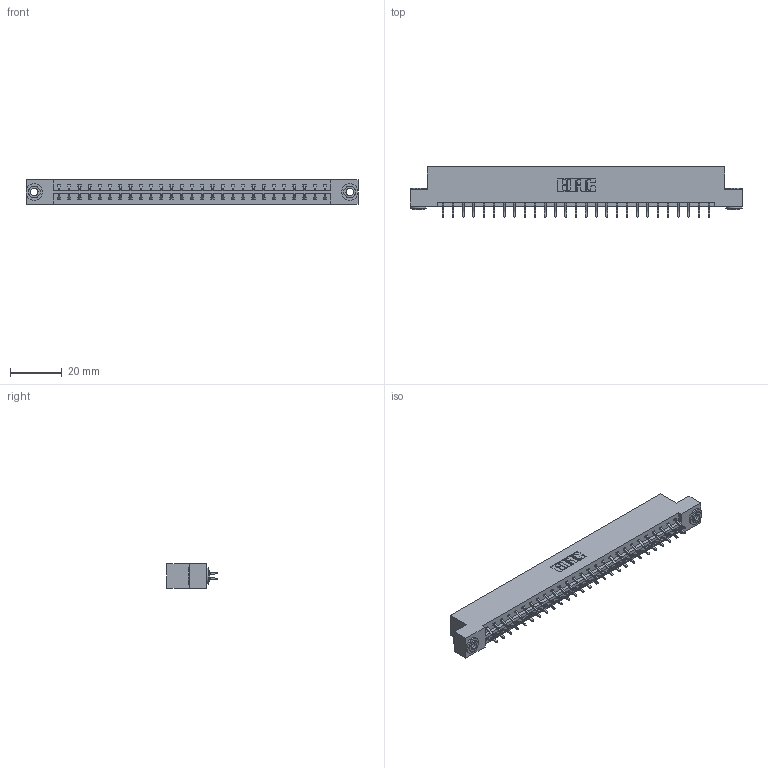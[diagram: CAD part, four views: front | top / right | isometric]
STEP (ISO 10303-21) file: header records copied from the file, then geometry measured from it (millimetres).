
FILE_DESCRIPTION (( 'STEP AP203' ), '1' );
FILE_NAME ('833-054-556-203.STEP', '2020-06-04T21:29:43', ( '' ), ( '' ), 'SwSTEP 2.0', 'SolidWorks 2020', '' );
FILE_SCHEMA (( 'CONFIG_CONTROL_DESIGN' ));
Length unit declared in the file: inch
Products named in the file (4): 345-292-001_556 Tail; 345-250-002_345-250-002-102; 833 Part_Flush - .156 Dia - TH; 833-054-556-203
Assembly tree (57 placements, depth 2):
  833-054-556-203
    833 Part_Flush - .156 Dia - TH
    345-292-001_556 Tail  x54
    345-250-002_345-250-002-102  x2
Bounding box: 128.52 x 19.57 x 9.4 mm (x, y, z)
Volume: 12998.5 mm3; surface area: 15374 mm2
Topology: 57 solids, 57 shells, 3284 faces, 9729 edges, 6410 vertices
Faces by surface type: plane 2240, cylinder 1036, cone 8
Entity records: 20180 total; most frequent: CARTESIAN_POINT 3353, ORIENTED_EDGE 3270, DIRECTION 2913, EDGE_CURVE 1635, VECTOR 1475, LINE 1475, VERTEX_POINT 1086, AXIS2_PLACEMENT_3D 719
